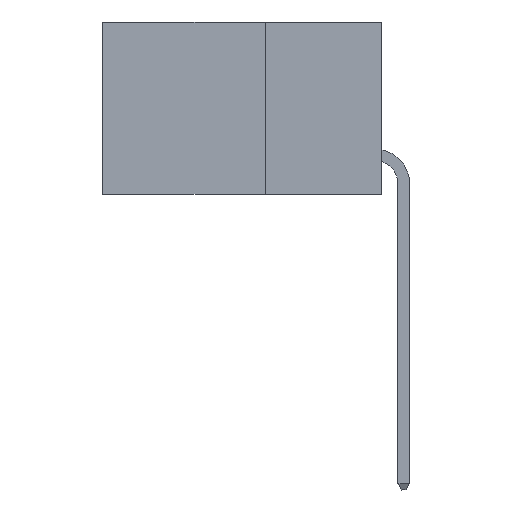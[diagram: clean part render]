
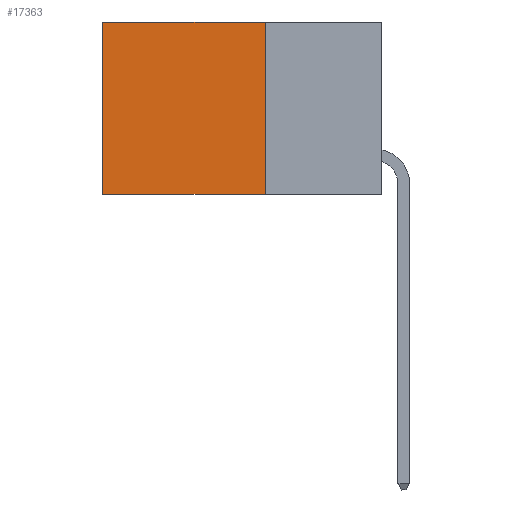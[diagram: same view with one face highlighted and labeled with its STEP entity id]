
A CAD part, left-side view. The second image highlights one B-rep face of the part: STEP entity #17363.
In plain terms, the highlighted planar face has unit normal (-1, 0, 0).
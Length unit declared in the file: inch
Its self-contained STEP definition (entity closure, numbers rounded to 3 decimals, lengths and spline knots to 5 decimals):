
#76 = CARTESIAN_POINT ( 'NONE',  ( 0.2875, 0.25, -0.37 ) ) ;
#4652 = CARTESIAN_POINT ( 'NONE',  ( 0.2875, 0.25, 0. ) ) ;
#4892 = VERTEX_POINT ( 'NONE', #33048 ) ;
#5392 = DIRECTION ( 'NONE',  ( 0., 1., 0. ) ) ;
#5612 = LINE ( 'NONE', #25661, #27770 ) ;
#7603 = DIRECTION ( 'NONE',  ( 0., 0., -1. ) ) ;
#8859 = ORIENTED_EDGE ( 'NONE', *, *, #11779, .F. ) ;
#8862 = EDGE_CURVE ( 'NONE', #15307, #30658, #5612, .T. ) ;
#10298 = EDGE_CURVE ( 'NONE', #30658, #4892, #12438, .T. ) ;
#11779 = EDGE_CURVE ( 'NONE', #15307, #16242, #22271, .T. ) ;
#12438 = LINE ( 'NONE', #27752, #19313 ) ;
#13835 = LINE ( 'NONE', #25219, #35571 ) ;
#15307 = VERTEX_POINT ( 'NONE', #16306 ) ;
#15573 = VECTOR ( 'NONE', #28504, 39.37008 ) ;
#16200 = ORIENTED_EDGE ( 'NONE', *, *, #8862, .T. ) ;
#16242 = VERTEX_POINT ( 'NONE', #76 ) ;
#16306 = CARTESIAN_POINT ( 'NONE',  ( 0.2875, 0.25, 0. ) ) ;
#16424 = DIRECTION ( 'NONE',  ( 0., 0., -1. ) ) ;
#17363 = ADVANCED_FACE ( 'NONE', ( #22738 ), #24713, .F. ) ;
#17756 = ORIENTED_EDGE ( 'NONE', *, *, #10298, .T. ) ;
#19313 = VECTOR ( 'NONE', #16424, 39.37008 ) ;
#19829 = EDGE_LOOP ( 'NONE', ( #17756, #32762, #8859, #16200 ) ) ;
#19988 = CARTESIAN_POINT ( 'NONE',  ( 0.2875, 0.25, 0. ) ) ;
#22271 = LINE ( 'NONE', #19988, #15573 ) ;
#22738 = FACE_OUTER_BOUND ( 'NONE', #19829, .T. ) ;
#24713 = PLANE ( 'NONE',  #31599 ) ;
#24791 = EDGE_CURVE ( 'NONE', #16242, #4892, #13835, .T. ) ;
#24961 = DIRECTION ( 'NONE',  ( 1., 0., 0. ) ) ;
#25219 = CARTESIAN_POINT ( 'NONE',  ( 0.2875, 0.25, -0.37 ) ) ;
#25661 = CARTESIAN_POINT ( 'NONE',  ( 0.2875, 0.25, 0. ) ) ;
#27752 = CARTESIAN_POINT ( 'NONE',  ( 0.2875, 0.6, 0. ) ) ;
#27770 = VECTOR ( 'NONE', #5392, 39.37008 ) ;
#27941 = DIRECTION ( 'NONE',  ( 0., 1., 0. ) ) ;
#28504 = DIRECTION ( 'NONE',  ( 0., 0., -1. ) ) ;
#29545 = CARTESIAN_POINT ( 'NONE',  ( 0.2875, 0.6, 0. ) ) ;
#30658 = VERTEX_POINT ( 'NONE', #29545 ) ;
#31599 = AXIS2_PLACEMENT_3D ( 'NONE', #4652, #24961, #7603 ) ;
#32762 = ORIENTED_EDGE ( 'NONE', *, *, #24791, .F. ) ;
#33048 = CARTESIAN_POINT ( 'NONE',  ( 0.2875, 0.6, -0.37 ) ) ;
#35571 = VECTOR ( 'NONE', #27941, 39.37008 ) ;
